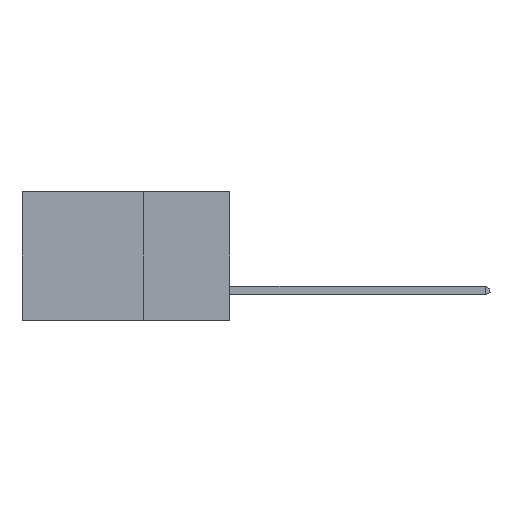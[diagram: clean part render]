
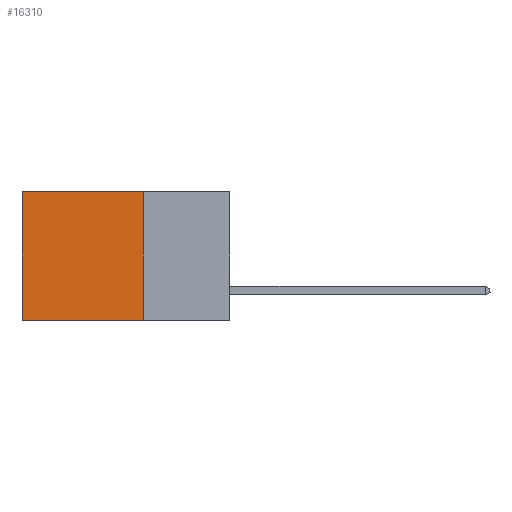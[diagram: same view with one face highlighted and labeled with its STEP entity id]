
A CAD part, left-side view. The second image highlights one B-rep face of the part: STEP entity #16310.
In plain terms, the highlighted planar face has unit normal (-1, 0, 0).
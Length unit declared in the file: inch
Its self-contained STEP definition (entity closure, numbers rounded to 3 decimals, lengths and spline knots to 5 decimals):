
#1170 = ORIENTED_EDGE ( 'NONE', *, *, #26385, .F. ) ;
#2000 = DIRECTION ( 'NONE',  ( 0., 0., -1. ) ) ;
#2606 = CARTESIAN_POINT ( 'NONE',  ( 0.298, 0.25, 0. ) ) ;
#3188 = ORIENTED_EDGE ( 'NONE', *, *, #17076, .T. ) ;
#3778 = VERTEX_POINT ( 'NONE', #25936 ) ;
#3905 = CARTESIAN_POINT ( 'NONE',  ( 0.298, 0.25, 0. ) ) ;
#3960 = VECTOR ( 'NONE', #22779, 39.37008 ) ;
#6089 = EDGE_CURVE ( 'NONE', #7140, #27152, #18408, .T. ) ;
#6233 = DIRECTION ( 'NONE',  ( 1., 0., 0. ) ) ;
#6846 = DIRECTION ( 'NONE',  ( 0., 0., -1. ) ) ;
#7140 = VERTEX_POINT ( 'NONE', #22018 ) ;
#8538 = VECTOR ( 'NONE', #28385, 39.37008 ) ;
#9027 = EDGE_CURVE ( 'NONE', #15745, #3778, #21401, .T. ) ;
#9144 = VECTOR ( 'NONE', #6846, 39.37008 ) ;
#10451 = DIRECTION ( 'NONE',  ( 0., 1., 0. ) ) ;
#11710 = LINE ( 'NONE', #15393, #29009 ) ;
#15027 = CARTESIAN_POINT ( 'NONE',  ( 0.298, 0.6, -0.37 ) ) ;
#15393 = CARTESIAN_POINT ( 'NONE',  ( 0.298, 0.25, -0.37 ) ) ;
#15745 = VERTEX_POINT ( 'NONE', #24995 ) ;
#15915 = CARTESIAN_POINT ( 'NONE',  ( 0.298, 0.6, 0. ) ) ;
#16188 = AXIS2_PLACEMENT_3D ( 'NONE', #3905, #6233, #2000 ) ;
#16310 = ADVANCED_FACE ( 'NONE', ( #17924 ), #22245, .F. ) ;
#17076 = EDGE_CURVE ( 'NONE', #15745, #7140, #18288, .T. ) ;
#17924 = FACE_OUTER_BOUND ( 'NONE', #27459, .T. ) ;
#18288 = LINE ( 'NONE', #23756, #8538 ) ;
#18408 = LINE ( 'NONE', #15915, #3960 ) ;
#18821 = ORIENTED_EDGE ( 'NONE', *, *, #9027, .F. ) ;
#21401 = LINE ( 'NONE', #2606, #9144 ) ;
#22018 = CARTESIAN_POINT ( 'NONE',  ( 0.298, 0.6, 0. ) ) ;
#22245 = PLANE ( 'NONE',  #16188 ) ;
#22779 = DIRECTION ( 'NONE',  ( 0., 0., -1. ) ) ;
#23756 = CARTESIAN_POINT ( 'NONE',  ( 0.298, 0.25, 0. ) ) ;
#24995 = CARTESIAN_POINT ( 'NONE',  ( 0.298, 0.25, 0. ) ) ;
#25936 = CARTESIAN_POINT ( 'NONE',  ( 0.298, 0.25, -0.37 ) ) ;
#26385 = EDGE_CURVE ( 'NONE', #3778, #27152, #11710, .T. ) ;
#27152 = VERTEX_POINT ( 'NONE', #15027 ) ;
#27459 = EDGE_LOOP ( 'NONE', ( #28617, #1170, #18821, #3188 ) ) ;
#28385 = DIRECTION ( 'NONE',  ( 0., 1., 0. ) ) ;
#28617 = ORIENTED_EDGE ( 'NONE', *, *, #6089, .T. ) ;
#29009 = VECTOR ( 'NONE', #10451, 39.37008 ) ;
